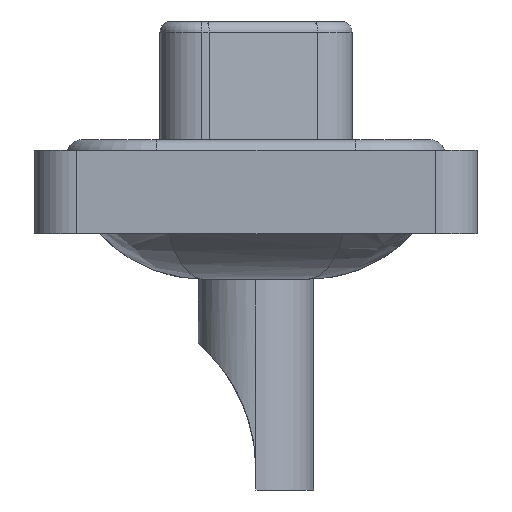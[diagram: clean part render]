
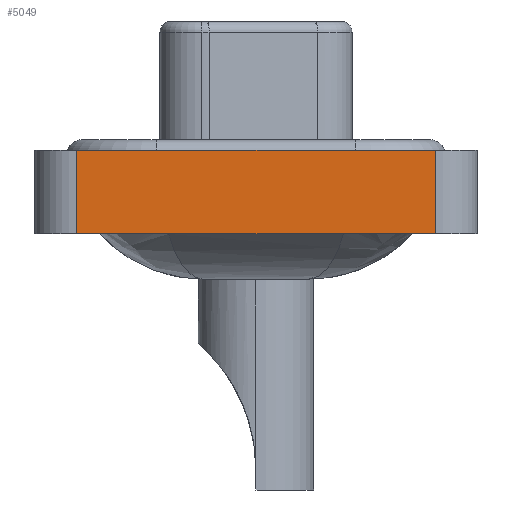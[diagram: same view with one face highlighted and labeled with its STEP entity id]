
A CAD part, left-side view. The second image highlights one B-rep face of the part: STEP entity #5049.
In plain terms, the highlighted planar face has unit normal (-1, 0, 0).
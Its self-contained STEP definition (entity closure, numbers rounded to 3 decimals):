
#191 = VECTOR ( 'NONE', #2210, 1000. ) ;
#2210 = DIRECTION ( 'NONE',  ( 0., -1., 0. ) ) ;
#2436 = VERTEX_POINT ( 'NONE', #2582 ) ;
#2582 = CARTESIAN_POINT ( 'NONE',  ( -7.35, 8.55, 0.4 ) ) ;
#2621 = ORIENTED_EDGE ( 'NONE', *, *, #14538, .F. ) ;
#3343 = LINE ( 'NONE', #10026, #14469 ) ;
#3803 = EDGE_CURVE ( 'NONE', #9565, #13788, #5023, .T. ) ;
#4614 = CARTESIAN_POINT ( 'NONE',  ( -7.35, -8.55, -3.6 ) ) ;
#4774 = DIRECTION ( 'NONE',  ( -1., 0., 0. ) ) ;
#5023 = LINE ( 'NONE', #16269, #5281 ) ;
#5049 = ADVANCED_FACE ( 'NONE', ( #15838 ), #17379, .T. ) ;
#5281 = VECTOR ( 'NONE', #7775, 1000. ) ;
#5336 = ORIENTED_EDGE ( 'NONE', *, *, #5657, .F. ) ;
#5657 = EDGE_CURVE ( 'NONE', #13615, #2436, #3343, .T. ) ;
#6059 = ORIENTED_EDGE ( 'NONE', *, *, #3803, .T. ) ;
#6338 = CARTESIAN_POINT ( 'NONE',  ( -7.35, -8.55, -3.6 ) ) ;
#7460 = DIRECTION ( 'NONE',  ( 0., 0., 1. ) ) ;
#7775 = DIRECTION ( 'NONE',  ( 0., 0., 1. ) ) ;
#9565 = VERTEX_POINT ( 'NONE', #4614 ) ;
#10026 = CARTESIAN_POINT ( 'NONE',  ( -7.35, 8.55, -3.6 ) ) ;
#10412 = EDGE_LOOP ( 'NONE', ( #6059, #2621, #5336, #12124 ) ) ;
#10770 = CARTESIAN_POINT ( 'NONE',  ( -7.35, -8.55, 0.4 ) ) ;
#12124 = ORIENTED_EDGE ( 'NONE', *, *, #14432, .T. ) ;
#12282 = CARTESIAN_POINT ( 'NONE',  ( -7.35, 8.55, -3.6 ) ) ;
#13247 = DIRECTION ( 'NONE',  ( 0., -1., 0. ) ) ;
#13615 = VERTEX_POINT ( 'NONE', #12282 ) ;
#13788 = VERTEX_POINT ( 'NONE', #16936 ) ;
#14049 = AXIS2_PLACEMENT_3D ( 'NONE', #6338, #4774, #17476 ) ;
#14432 = EDGE_CURVE ( 'NONE', #13615, #9565, #15995, .T. ) ;
#14469 = VECTOR ( 'NONE', #7460, 1000. ) ;
#14538 = EDGE_CURVE ( 'NONE', #2436, #13788, #16169, .T. ) ;
#14728 = VECTOR ( 'NONE', #13247, 1000. ) ;
#15725 = CARTESIAN_POINT ( 'NONE',  ( -7.35, -8.55, -3.6 ) ) ;
#15838 = FACE_OUTER_BOUND ( 'NONE', #10412, .T. ) ;
#15995 = LINE ( 'NONE', #15725, #14728 ) ;
#16169 = LINE ( 'NONE', #10770, #191 ) ;
#16269 = CARTESIAN_POINT ( 'NONE',  ( -7.35, -8.55, -3.6 ) ) ;
#16936 = CARTESIAN_POINT ( 'NONE',  ( -7.35, -8.55, 0.4 ) ) ;
#17379 = PLANE ( 'NONE',  #14049 ) ;
#17476 = DIRECTION ( 'NONE',  ( 0., 0., 1. ) ) ;
